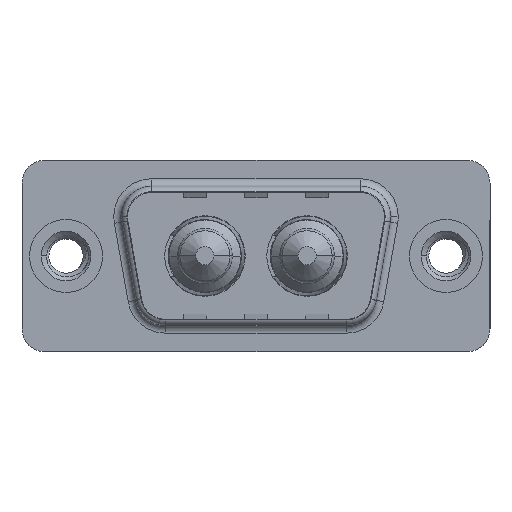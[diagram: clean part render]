
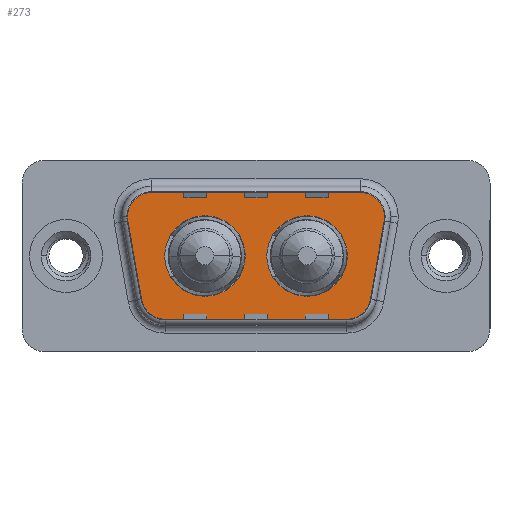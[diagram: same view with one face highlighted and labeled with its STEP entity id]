
A CAD part, top view. The second image highlights one B-rep face of the part: STEP entity #273.
In plain terms, the highlighted planar face has unit normal (0, 0, 1).
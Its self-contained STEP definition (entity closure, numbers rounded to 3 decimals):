
#5 = CARTESIAN_POINT ( 'NONE',  ( 9.14, 0., 0. ) ) ;
#13 = EDGE_CURVE ( 'NONE', #6144, #9933, #9461, .T. ) ;
#69 = PLANE ( 'NONE',  #845 ) ;
#273 = ADVANCED_FACE ( 'NONE', ( #12130, #2396, #7360 ), #69, .T. ) ;
#562 = CARTESIAN_POINT ( 'NONE',  ( 6.49, 0., 0. ) ) ;
#602 = VECTOR ( 'NONE', #9283, 1000. ) ;
#643 = CARTESIAN_POINT ( 'NONE',  ( 18.541, -2.9, 0. ) ) ;
#711 = CIRCLE ( 'NONE', #3218, 2. ) ;
#726 = DIRECTION ( 'NONE',  ( 1., 0., 0. ) ) ;
#836 = CARTESIAN_POINT ( 'NONE',  ( 13.21, 0., 0. ) ) ;
#845 = AXIS2_PLACEMENT_3D ( 'NONE', #643, #7399, #9939 ) ;
#946 = DIRECTION ( 'NONE',  ( 1., 0., 0. ) ) ;
#981 = CIRCLE ( 'NONE', #10139, 2.65 ) ;
#1042 = AXIS2_PLACEMENT_3D ( 'NONE', #8441, #2826, #9413 ) ;
#1161 = VERTEX_POINT ( 'NONE', #1377 ) ;
#1377 = CARTESIAN_POINT ( 'NONE',  ( 4.489, -3.247, 0. ) ) ;
#1540 = ORIENTED_EDGE ( 'NONE', *, *, #10740, .T. ) ;
#1573 = AXIS2_PLACEMENT_3D ( 'NONE', #1576, #2167, #11513 ) ;
#1576 = CARTESIAN_POINT ( 'NONE',  ( 19.564, 2.9, 0. ) ) ;
#1806 = CIRCLE ( 'NONE', #6686, 2.65 ) ;
#2063 = EDGE_LOOP ( 'NONE', ( #8403, #4889 ) ) ;
#2136 = CARTESIAN_POINT ( 'NONE',  ( 6.459, -4.9, 0. ) ) ;
#2153 = CIRCLE ( 'NONE', #1042, 2. ) ;
#2167 = DIRECTION ( 'NONE',  ( 0., 0., 1. ) ) ;
#2233 = VERTEX_POINT ( 'NONE', #8098 ) ;
#2283 = ORIENTED_EDGE ( 'NONE', *, *, #8875, .T. ) ;
#2396 = FACE_BOUND ( 'NONE', #2063, .T. ) ;
#2460 = VERTEX_POINT ( 'NONE', #3026 ) ;
#2509 = DIRECTION ( 'NONE',  ( 0., 0., 1. ) ) ;
#2539 = DIRECTION ( 'NONE',  ( 0., 0., 1. ) ) ;
#2826 = DIRECTION ( 'NONE',  ( 0., 0., 1. ) ) ;
#2983 = ORIENTED_EDGE ( 'NONE', *, *, #4356, .T. ) ;
#3026 = CARTESIAN_POINT ( 'NONE',  ( 21.534, 2.553, 0. ) ) ;
#3036 = VECTOR ( 'NONE', #8124, 1000. ) ;
#3201 = CARTESIAN_POINT ( 'NONE',  ( 18.51, 0., 0. ) ) ;
#3218 = AXIS2_PLACEMENT_3D ( 'NONE', #10298, #10307, #6700 ) ;
#3394 = CIRCLE ( 'NONE', #1573, 2. ) ;
#3547 = CARTESIAN_POINT ( 'NONE',  ( 20.511, -3.247, 0. ) ) ;
#3626 = CARTESIAN_POINT ( 'NONE',  ( 3.466, 2.553, 0. ) ) ;
#3664 = CARTESIAN_POINT ( 'NONE',  ( 3.466, 2.553, 0. ) ) ;
#3710 = CARTESIAN_POINT ( 'NONE',  ( 18.541, -2.9, 0. ) ) ;
#3738 = DIRECTION ( 'NONE',  ( 0., 0., 1. ) ) ;
#3864 = EDGE_CURVE ( 'NONE', #6439, #2233, #711, .T. ) ;
#4338 = VECTOR ( 'NONE', #11494, 1000. ) ;
#4356 = EDGE_CURVE ( 'NONE', #9933, #4997, #11291, .T. ) ;
#4607 = ORIENTED_EDGE ( 'NONE', *, *, #5552, .F. ) ;
#4793 = EDGE_LOOP ( 'NONE', ( #4607, #8920 ) ) ;
#4876 = AXIS2_PLACEMENT_3D ( 'NONE', #8117, #2509, #9075 ) ;
#4889 = ORIENTED_EDGE ( 'NONE', *, *, #7223, .F. ) ;
#4997 = VERTEX_POINT ( 'NONE', #3547 ) ;
#5110 = ORIENTED_EDGE ( 'NONE', *, *, #6678, .T. ) ;
#5309 = EDGE_CURVE ( 'NONE', #1161, #6144, #7966, .T. ) ;
#5552 = EDGE_CURVE ( 'NONE', #7427, #9956, #9007, .T. ) ;
#5761 = CARTESIAN_POINT ( 'NONE',  ( 21.534, 2.553, 0. ) ) ;
#6117 = CARTESIAN_POINT ( 'NONE',  ( 6.459, -2.9, 0. ) ) ;
#6144 = VERTEX_POINT ( 'NONE', #2136 ) ;
#6365 = DIRECTION ( 'NONE',  ( 0., 0., 1. ) ) ;
#6439 = VERTEX_POINT ( 'NONE', #10762 ) ;
#6457 = DIRECTION ( 'NONE',  ( 0., 0., 1. ) ) ;
#6678 = EDGE_CURVE ( 'NONE', #2460, #6439, #3394, .T. ) ;
#6686 = AXIS2_PLACEMENT_3D ( 'NONE', #8146, #2539, #9108 ) ;
#6700 = DIRECTION ( 'NONE',  ( -1., 0., 0. ) ) ;
#6898 = VECTOR ( 'NONE', #8941, 1000. ) ;
#7223 = EDGE_CURVE ( 'NONE', #10994, #8250, #1806, .T. ) ;
#7280 = CARTESIAN_POINT ( 'NONE',  ( 18.541, -4.9, 0. ) ) ;
#7360 = FACE_OUTER_BOUND ( 'NONE', #9738, .T. ) ;
#7399 = DIRECTION ( 'NONE',  ( 0., 0., 1. ) ) ;
#7427 = VERTEX_POINT ( 'NONE', #3201 ) ;
#7646 = CARTESIAN_POINT ( 'NONE',  ( 11.79, 0., 0. ) ) ;
#7665 = ORIENTED_EDGE ( 'NONE', *, *, #8486, .T. ) ;
#7801 = DIRECTION ( 'NONE',  ( 0., 0., 1. ) ) ;
#7966 = CIRCLE ( 'NONE', #11878, 2. ) ;
#7978 = VERTEX_POINT ( 'NONE', #12123 ) ;
#8098 = CARTESIAN_POINT ( 'NONE',  ( 19.564, 4.9, 0. ) ) ;
#8117 = CARTESIAN_POINT ( 'NONE',  ( 15.86, 0., 0. ) ) ;
#8124 = DIRECTION ( 'NONE',  ( -1., 0., 0. ) ) ;
#8146 = CARTESIAN_POINT ( 'NONE',  ( 9.14, 0., 0. ) ) ;
#8250 = VERTEX_POINT ( 'NONE', #7646 ) ;
#8333 = LINE ( 'NONE', #3626, #602 ) ;
#8403 = ORIENTED_EDGE ( 'NONE', *, *, #11998, .F. ) ;
#8441 = CARTESIAN_POINT ( 'NONE',  ( 5.436, 2.9, 0. ) ) ;
#8486 = EDGE_CURVE ( 'NONE', #4997, #2460, #9404, .T. ) ;
#8712 = CIRCLE ( 'NONE', #4876, 2.65 ) ;
#8721 = CARTESIAN_POINT ( 'NONE',  ( 15.86, 0., 0. ) ) ;
#8749 = AXIS2_PLACEMENT_3D ( 'NONE', #3710, #3738, #9309 ) ;
#8875 = EDGE_CURVE ( 'NONE', #8919, #1161, #8333, .T. ) ;
#8916 = ORIENTED_EDGE ( 'NONE', *, *, #9428, .T. ) ;
#8919 = VERTEX_POINT ( 'NONE', #3664 ) ;
#8920 = ORIENTED_EDGE ( 'NONE', *, *, #11384, .F. ) ;
#8941 = DIRECTION ( 'NONE',  ( 1., 0., 0. ) ) ;
#8997 = CARTESIAN_POINT ( 'NONE',  ( 5.436, 4.9, 0. ) ) ;
#9007 = CIRCLE ( 'NONE', #11646, 2.65 ) ;
#9075 = DIRECTION ( 'NONE',  ( 1., 0., 0. ) ) ;
#9101 = DIRECTION ( 'NONE',  ( -1., 0., 0. ) ) ;
#9108 = DIRECTION ( 'NONE',  ( 1., 0., 0. ) ) ;
#9283 = DIRECTION ( 'NONE',  ( 0.174, -0.985, 0. ) ) ;
#9309 = DIRECTION ( 'NONE',  ( 1., 0., 0. ) ) ;
#9404 = LINE ( 'NONE', #5761, #4338 ) ;
#9413 = DIRECTION ( 'NONE',  ( 1., 0., 0. ) ) ;
#9428 = EDGE_CURVE ( 'NONE', #2233, #7978, #10568, .T. ) ;
#9461 = LINE ( 'NONE', #11573, #6898 ) ;
#9738 = EDGE_LOOP ( 'NONE', ( #2983, #7665, #5110, #11253, #8916, #1540, #2283, #9969, #11468 ) ) ;
#9933 = VERTEX_POINT ( 'NONE', #7280 ) ;
#9939 = DIRECTION ( 'NONE',  ( 1., 0., 0. ) ) ;
#9956 = VERTEX_POINT ( 'NONE', #836 ) ;
#9969 = ORIENTED_EDGE ( 'NONE', *, *, #5309, .T. ) ;
#10139 = AXIS2_PLACEMENT_3D ( 'NONE', #5, #6457, #946 ) ;
#10298 = CARTESIAN_POINT ( 'NONE',  ( 19.564, 2.9, 0. ) ) ;
#10307 = DIRECTION ( 'NONE',  ( 0., 0., 1. ) ) ;
#10568 = LINE ( 'NONE', #8997, #3036 ) ;
#10740 = EDGE_CURVE ( 'NONE', #7978, #8919, #2153, .T. ) ;
#10762 = CARTESIAN_POINT ( 'NONE',  ( 21.564, 2.9, 0. ) ) ;
#10994 = VERTEX_POINT ( 'NONE', #562 ) ;
#11253 = ORIENTED_EDGE ( 'NONE', *, *, #3864, .T. ) ;
#11291 = CIRCLE ( 'NONE', #8749, 2. ) ;
#11384 = EDGE_CURVE ( 'NONE', #9956, #7427, #8712, .T. ) ;
#11468 = ORIENTED_EDGE ( 'NONE', *, *, #13, .T. ) ;
#11494 = DIRECTION ( 'NONE',  ( 0.174, 0.985, 0. ) ) ;
#11513 = DIRECTION ( 'NONE',  ( -1., 0., 0. ) ) ;
#11573 = CARTESIAN_POINT ( 'NONE',  ( 6.459, -4.9, 0. ) ) ;
#11646 = AXIS2_PLACEMENT_3D ( 'NONE', #8721, #7801, #726 ) ;
#11878 = AXIS2_PLACEMENT_3D ( 'NONE', #6117, #6365, #9101 ) ;
#11998 = EDGE_CURVE ( 'NONE', #8250, #10994, #981, .T. ) ;
#12123 = CARTESIAN_POINT ( 'NONE',  ( 5.436, 4.9, 0. ) ) ;
#12130 = FACE_BOUND ( 'NONE', #4793, .T. ) ;
